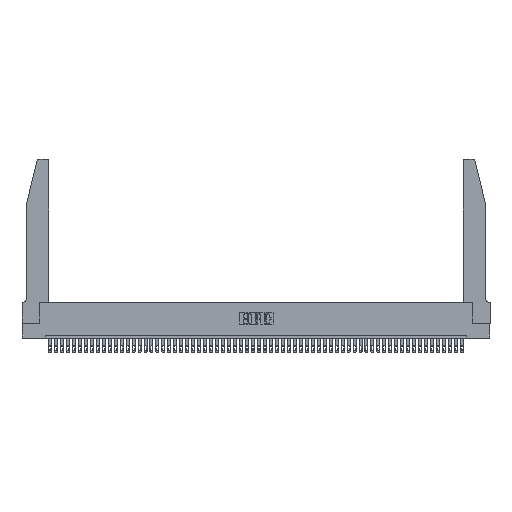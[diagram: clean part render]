
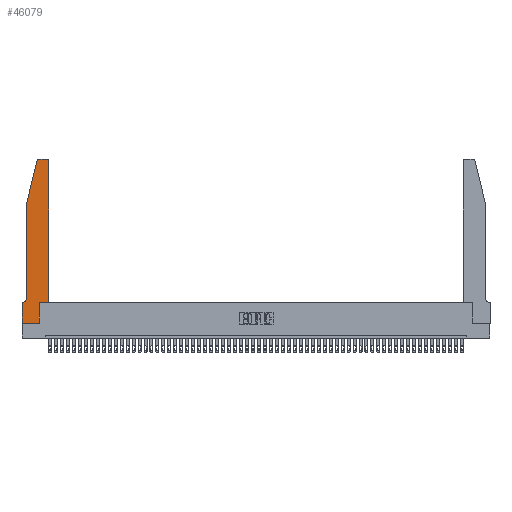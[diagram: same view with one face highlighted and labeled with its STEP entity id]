
A CAD part, top view. The second image highlights one B-rep face of the part: STEP entity #46079.
In plain terms, the highlighted planar face has unit normal (0, 0, 1).
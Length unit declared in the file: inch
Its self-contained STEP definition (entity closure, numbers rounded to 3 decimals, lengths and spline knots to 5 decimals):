
#87 = EDGE_CURVE ( 'NONE', #5621, #47509, #51920, .T. ) ;
#809 = EDGE_CURVE ( 'NONE', #19035, #12804, #5221, .T. ) ;
#2115 = DIRECTION ( 'NONE',  ( 1., 0., 0. ) ) ;
#2600 = VECTOR ( 'NONE', #47859, 39.37008 ) ;
#3461 = VECTOR ( 'NONE', #11534, 39.37008 ) ;
#3980 = AXIS2_PLACEMENT_3D ( 'NONE', #24086, #49013, #28440 ) ;
#5221 = LINE ( 'NONE', #29539, #7264 ) ;
#5430 = EDGE_CURVE ( 'NONE', #12449, #53396, #15229, .T. ) ;
#5621 = VERTEX_POINT ( 'NONE', #19730 ) ;
#6205 = CIRCLE ( 'NONE', #41109, 0.07 ) ;
#6337 = CARTESIAN_POINT ( 'NONE',  ( 0.284, 2.72, 0.37 ) ) ;
#6667 = CARTESIAN_POINT ( 'NONE',  ( 0.2865, 0.35, 0.37 ) ) ;
#7009 = CARTESIAN_POINT ( 'NONE',  ( 0.2865, 0., 0.37 ) ) ;
#7264 = VECTOR ( 'NONE', #45798, 39.37008 ) ;
#7543 = CARTESIAN_POINT ( 'NONE',  ( 0., 0., 0.37 ) ) ;
#7772 = ORIENTED_EDGE ( 'NONE', *, *, #8910, .T. ) ;
#7822 = ORIENTED_EDGE ( 'NONE', *, *, #25536, .T. ) ;
#7955 = PLANE ( 'NONE',  #41954 ) ;
#8117 = VERTEX_POINT ( 'NONE', #26185 ) ;
#8609 = LINE ( 'NONE', #40232, #9188 ) ;
#8786 = DIRECTION ( 'NONE',  ( -1., 0., 0. ) ) ;
#8910 = EDGE_CURVE ( 'NONE', #33912, #12449, #51167, .T. ) ;
#8955 = ORIENTED_EDGE ( 'NONE', *, *, #36147, .T. ) ;
#9188 = VECTOR ( 'NONE', #15676, 39.37008 ) ;
#10017 = LINE ( 'NONE', #10727, #34549 ) ;
#10075 = EDGE_CURVE ( 'NONE', #34199, #33912, #21340, .T. ) ;
#10727 = CARTESIAN_POINT ( 'NONE',  ( 0.4505, 0.35, 0.37 ) ) ;
#10911 = VERTEX_POINT ( 'NONE', #44273 ) ;
#11264 = ORIENTED_EDGE ( 'NONE', *, *, #13053, .T. ) ;
#11410 = DIRECTION ( 'NONE',  ( 0., 0., 1. ) ) ;
#11534 = DIRECTION ( 'NONE',  ( 1., 0., 0. ) ) ;
#12086 = CARTESIAN_POINT ( 'NONE',  ( 0.4505, 0.35, 0.37 ) ) ;
#12449 = VERTEX_POINT ( 'NONE', #7009 ) ;
#12804 = VERTEX_POINT ( 'NONE', #42804 ) ;
#12941 = AXIS2_PLACEMENT_3D ( 'NONE', #6337, #14284, #47306 ) ;
#13053 = EDGE_CURVE ( 'NONE', #12804, #8117, #6205, .T. ) ;
#13357 = CARTESIAN_POINT ( 'NONE',  ( 0., 0., 0.37 ) ) ;
#14282 = DIRECTION ( 'NONE',  ( 0., 1., 0. ) ) ;
#14284 = DIRECTION ( 'NONE',  ( 0., 0., 1. ) ) ;
#15228 = ORIENTED_EDGE ( 'NONE', *, *, #5430, .T. ) ;
#15229 = LINE ( 'NONE', #6667, #42284 ) ;
#15676 = DIRECTION ( 'NONE',  ( -1., 0., 0. ) ) ;
#15849 = VECTOR ( 'NONE', #8786, 39.37008 ) ;
#17084 = DIRECTION ( 'NONE',  ( 0., 1., 0. ) ) ;
#19035 = VERTEX_POINT ( 'NONE', #36364 ) ;
#19541 = ORIENTED_EDGE ( 'NONE', *, *, #10075, .T. ) ;
#19730 = CARTESIAN_POINT ( 'NONE',  ( 0.4505, 2.72, 0.37 ) ) ;
#20125 = EDGE_CURVE ( 'NONE', #47509, #36502, #8609, .T. ) ;
#20829 = FACE_OUTER_BOUND ( 'NONE', #39411, .T. ) ;
#21340 = LINE ( 'NONE', #13357, #2600 ) ;
#21488 = ORIENTED_EDGE ( 'NONE', *, *, #21865, .T. ) ;
#21637 = CARTESIAN_POINT ( 'NONE',  ( 0.4205, 2.75, 0.37 ) ) ;
#21865 = EDGE_CURVE ( 'NONE', #8117, #34199, #26738, .T. ) ;
#24086 = CARTESIAN_POINT ( 'NONE',  ( 0.4205, 2.72, 0.37 ) ) ;
#24598 = CARTESIAN_POINT ( 'NONE',  ( 0.284, 2.75, 0.37 ) ) ;
#25536 = EDGE_CURVE ( 'NONE', #53396, #10911, #40708, .T. ) ;
#25559 = CARTESIAN_POINT ( 'NONE',  ( 0.0755, 2., 0.37 ) ) ;
#26185 = CARTESIAN_POINT ( 'NONE',  ( 0.0055, 0.35, 0.37 ) ) ;
#26738 = LINE ( 'NONE', #28883, #15849 ) ;
#27042 = VECTOR ( 'NONE', #2115, 39.37008 ) ;
#27306 = CARTESIAN_POINT ( 'NONE',  ( 0.0055, 0.42, 0.37 ) ) ;
#28440 = DIRECTION ( 'NONE',  ( 1., 0., 0. ) ) ;
#28883 = CARTESIAN_POINT ( 'NONE',  ( 0.0755, 0.35, 0.37 ) ) ;
#29539 = CARTESIAN_POINT ( 'NONE',  ( 0.0755, 2., 0.37 ) ) ;
#30671 = CARTESIAN_POINT ( 'NONE',  ( 0.2865, 0.35, 0.37 ) ) ;
#33912 = VERTEX_POINT ( 'NONE', #52432 ) ;
#34199 = VERTEX_POINT ( 'NONE', #39058 ) ;
#34549 = VECTOR ( 'NONE', #14282, 39.37008 ) ;
#34695 = EDGE_CURVE ( 'NONE', #36502, #43665, #53003, .T. ) ;
#36147 = EDGE_CURVE ( 'NONE', #10911, #5621, #10017, .T. ) ;
#36364 = CARTESIAN_POINT ( 'NONE',  ( 0.0755, 2., 0.37 ) ) ;
#36502 = VERTEX_POINT ( 'NONE', #24598 ) ;
#36838 = DIRECTION ( 'NONE',  ( 1., 0., 0. ) ) ;
#38051 = ORIENTED_EDGE ( 'NONE', *, *, #87, .T. ) ;
#38784 = EDGE_CURVE ( 'NONE', #43665, #19035, #44013, .T. ) ;
#39058 = CARTESIAN_POINT ( 'NONE',  ( 0., 0.35, 0.37 ) ) ;
#39411 = EDGE_LOOP ( 'NONE', ( #49998, #53347, #50731, #47418, #11264, #21488, #19541, #7772, #15228, #7822, #8955, #38051 ) ) ;
#40232 = CARTESIAN_POINT ( 'NONE',  ( 0.2605, 2.75, 0.37 ) ) ;
#40463 = CARTESIAN_POINT ( 'NONE',  ( 0., 0.35, 0.37 ) ) ;
#40708 = LINE ( 'NONE', #12086, #27042 ) ;
#41109 = AXIS2_PLACEMENT_3D ( 'NONE', #27306, #43334, #51442 ) ;
#41766 = CARTESIAN_POINT ( 'NONE',  ( 0.25487, 2.72718, 0.37 ) ) ;
#41954 = AXIS2_PLACEMENT_3D ( 'NONE', #40463, #11410, #36838 ) ;
#42284 = VECTOR ( 'NONE', #17084, 39.37008 ) ;
#42804 = CARTESIAN_POINT ( 'NONE',  ( 0.0755, 0.42, 0.37 ) ) ;
#43334 = DIRECTION ( 'NONE',  ( 0., 0., -1. ) ) ;
#43665 = VERTEX_POINT ( 'NONE', #41766 ) ;
#44013 = LINE ( 'NONE', #25559, #50410 ) ;
#44273 = CARTESIAN_POINT ( 'NONE',  ( 0.4505, 0.35, 0.37 ) ) ;
#45798 = DIRECTION ( 'NONE',  ( 0., -1., 0. ) ) ;
#46079 = ADVANCED_FACE ( 'NONE', ( #20829 ), #7955, .T. ) ;
#46466 = DIRECTION ( 'NONE',  ( -0.239, -0.971, 0. ) ) ;
#47306 = DIRECTION ( 'NONE',  ( 1., 0., 0. ) ) ;
#47418 = ORIENTED_EDGE ( 'NONE', *, *, #809, .T. ) ;
#47509 = VERTEX_POINT ( 'NONE', #21637 ) ;
#47859 = DIRECTION ( 'NONE',  ( 0., -1., 0. ) ) ;
#49013 = DIRECTION ( 'NONE',  ( 0., 0., 1. ) ) ;
#49998 = ORIENTED_EDGE ( 'NONE', *, *, #20125, .T. ) ;
#50410 = VECTOR ( 'NONE', #46466, 39.37008 ) ;
#50731 = ORIENTED_EDGE ( 'NONE', *, *, #38784, .T. ) ;
#51167 = LINE ( 'NONE', #7543, #3461 ) ;
#51442 = DIRECTION ( 'NONE',  ( -1., 0., 0. ) ) ;
#51920 = CIRCLE ( 'NONE', #3980, 0.03 ) ;
#52432 = CARTESIAN_POINT ( 'NONE',  ( 0., 0., 0.37 ) ) ;
#53003 = CIRCLE ( 'NONE', #12941, 0.03 ) ;
#53347 = ORIENTED_EDGE ( 'NONE', *, *, #34695, .T. ) ;
#53396 = VERTEX_POINT ( 'NONE', #30671 ) ;
